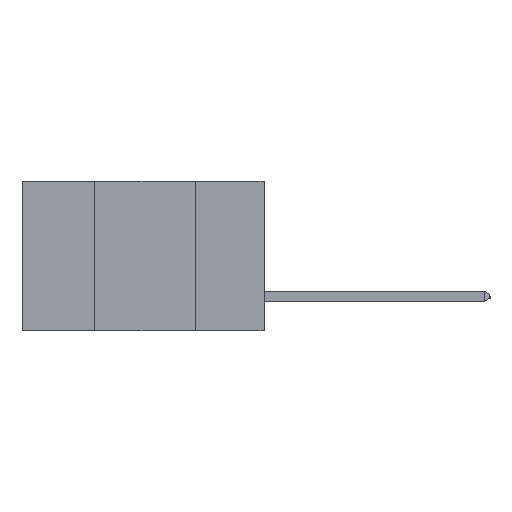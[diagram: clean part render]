
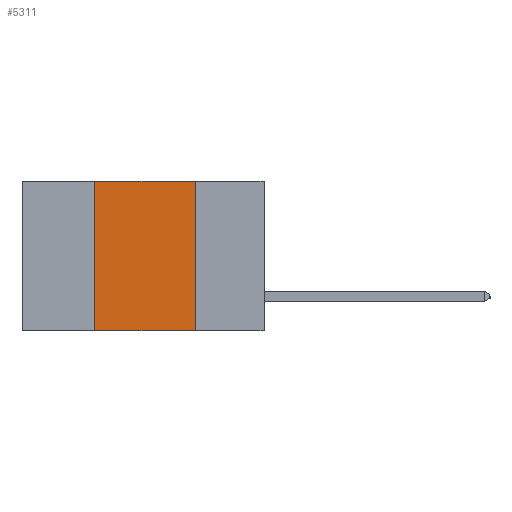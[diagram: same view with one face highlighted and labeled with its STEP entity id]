
A CAD part, left-side view. The second image highlights one B-rep face of the part: STEP entity #5311.
In plain terms, the highlighted planar face has unit normal (-1, 0, 0).
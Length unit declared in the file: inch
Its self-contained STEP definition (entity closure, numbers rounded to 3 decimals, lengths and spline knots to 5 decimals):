
#153 = DIRECTION ( 'NONE',  ( 0., 0., 1. ) ) ;
#655 = DIRECTION ( 'NONE',  ( 0., 0., -1. ) ) ;
#1575 = VECTOR ( 'NONE', #11434, 39.37008 ) ;
#2946 = CARTESIAN_POINT ( 'NONE',  ( 0., 0.17, 0. ) ) ;
#3401 = CARTESIAN_POINT ( 'NONE',  ( 0., 0.6, 0. ) ) ;
#3961 = ORIENTED_EDGE ( 'NONE', *, *, #9500, .F. ) ;
#4384 = VECTOR ( 'NONE', #11912, 39.37008 ) ;
#4566 = EDGE_CURVE ( 'NONE', #6326, #17411, #12402, .T. ) ;
#4636 = LINE ( 'NONE', #13695, #8332 ) ;
#4812 = VERTEX_POINT ( 'NONE', #2946 ) ;
#5262 = LINE ( 'NONE', #19101, #1575 ) ;
#5311 = ADVANCED_FACE ( 'NONE', ( #11230 ), #5712, .F. ) ;
#5712 = PLANE ( 'NONE',  #6428 ) ;
#6326 = VERTEX_POINT ( 'NONE', #13381 ) ;
#6428 = AXIS2_PLACEMENT_3D ( 'NONE', #3401, #6532, #655 ) ;
#6532 = DIRECTION ( 'NONE',  ( 1., 0., 0. ) ) ;
#7323 = DIRECTION ( 'NONE',  ( 0., -1., 0. ) ) ;
#8243 = CARTESIAN_POINT ( 'NONE',  ( 0., 0.6, -0.37 ) ) ;
#8332 = VECTOR ( 'NONE', #7323, 39.37008 ) ;
#9320 = CARTESIAN_POINT ( 'NONE',  ( 0., 0.42, 0. ) ) ;
#9500 = EDGE_CURVE ( 'NONE', #4812, #17411, #5262, .T. ) ;
#9656 = CARTESIAN_POINT ( 'NONE',  ( 0., 0.42, 0. ) ) ;
#11230 = FACE_OUTER_BOUND ( 'NONE', #17362, .T. ) ;
#11434 = DIRECTION ( 'NONE',  ( 0., 0., -1. ) ) ;
#11859 = VERTEX_POINT ( 'NONE', #9320 ) ;
#11912 = DIRECTION ( 'NONE',  ( 0., -1., 0. ) ) ;
#12402 = LINE ( 'NONE', #8243, #4384 ) ;
#12816 = CARTESIAN_POINT ( 'NONE',  ( 0., 0.17, -0.37 ) ) ;
#12967 = ORIENTED_EDGE ( 'NONE', *, *, #15901, .F. ) ;
#13381 = CARTESIAN_POINT ( 'NONE',  ( 0., 0.42, -0.37 ) ) ;
#13695 = CARTESIAN_POINT ( 'NONE',  ( 0., 0.6, 0. ) ) ;
#15901 = EDGE_CURVE ( 'NONE', #11859, #4812, #4636, .T. ) ;
#17084 = ORIENTED_EDGE ( 'NONE', *, *, #19284, .F. ) ;
#17362 = EDGE_LOOP ( 'NONE', ( #3961, #12967, #17084, #17560 ) ) ;
#17411 = VERTEX_POINT ( 'NONE', #12816 ) ;
#17560 = ORIENTED_EDGE ( 'NONE', *, *, #4566, .T. ) ;
#17699 = LINE ( 'NONE', #9656, #18170 ) ;
#18170 = VECTOR ( 'NONE', #153, 39.37008 ) ;
#19101 = CARTESIAN_POINT ( 'NONE',  ( 0., 0.17, 0. ) ) ;
#19284 = EDGE_CURVE ( 'NONE', #6326, #11859, #17699, .T. ) ;
